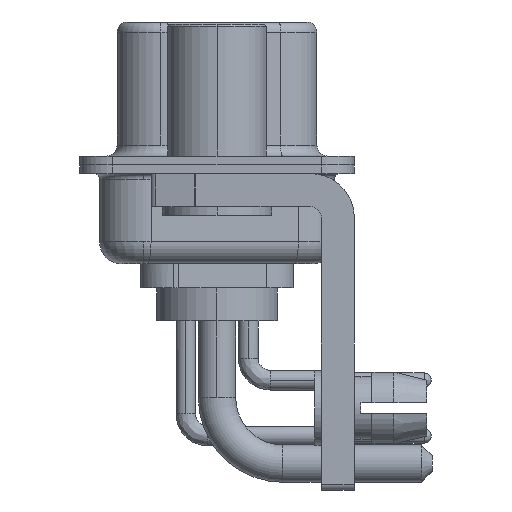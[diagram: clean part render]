
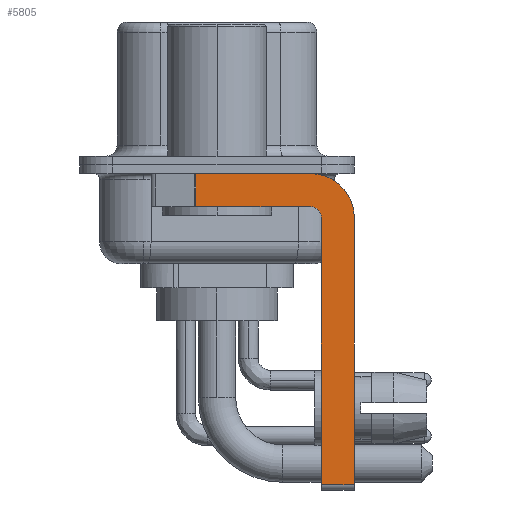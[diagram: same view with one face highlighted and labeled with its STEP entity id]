
A CAD part, left-side view. The second image highlights one B-rep face of the part: STEP entity #5805.
In plain terms, the highlighted planar face has unit normal (-1, 0, 0).
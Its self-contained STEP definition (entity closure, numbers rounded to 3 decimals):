
#283 = CARTESIAN_POINT ( 'NONE',  ( -2.9, -4.25, -1.9 ) ) ;
#370 = AXIS2_PLACEMENT_3D ( 'NONE', #6989, #23847, #5135 ) ;
#701 = EDGE_LOOP ( 'NONE', ( #30869, #20856, #23458, #31140, #3520, #12303, #23858, #1163 ) ) ;
#792 = VECTOR ( 'NONE', #8494, 1000. ) ;
#1113 = LINE ( 'NONE', #6142, #18823 ) ;
#1163 = ORIENTED_EDGE ( 'NONE', *, *, #11047, .F. ) ;
#1188 = AXIS2_PLACEMENT_3D ( 'NONE', #22629, #5762, #15649 ) ;
#1211 = CARTESIAN_POINT ( 'NONE',  ( -2.9, -4.75, -2.4 ) ) ;
#1866 = EDGE_CURVE ( 'NONE', #26353, #20936, #12810, .T. ) ;
#2112 = EDGE_CURVE ( 'NONE', #27599, #7513, #30706, .T. ) ;
#2295 = VECTOR ( 'NONE', #22790, 1000. ) ;
#3507 = VERTEX_POINT ( 'NONE', #7962 ) ;
#3520 = ORIENTED_EDGE ( 'NONE', *, *, #12509, .F. ) ;
#4243 = VERTEX_POINT ( 'NONE', #29832 ) ;
#5135 = DIRECTION ( 'NONE',  ( 0., 0., 1. ) ) ;
#5376 = AXIS2_PLACEMENT_3D ( 'NONE', #12757, #8661, #26011 ) ;
#5597 = CARTESIAN_POINT ( 'NONE',  ( -2.9, -4.25, -0.4 ) ) ;
#5762 = DIRECTION ( 'NONE',  ( 1., 0., 0. ) ) ;
#5805 = ADVANCED_FACE ( 'NONE', ( #27972 ), #24917, .F. ) ;
#6060 = CARTESIAN_POINT ( 'NONE',  ( -2.9, -4.25, -14.55 ) ) ;
#6142 = CARTESIAN_POINT ( 'NONE',  ( -2.9, -4.25, -1.9 ) ) ;
#6989 = CARTESIAN_POINT ( 'NONE',  ( -2.9, -4.25, -2.4 ) ) ;
#7513 = VERTEX_POINT ( 'NONE', #13481 ) ;
#7633 = CARTESIAN_POINT ( 'NONE',  ( -2.9, -6.25, -2.4 ) ) ;
#7962 = CARTESIAN_POINT ( 'NONE',  ( -2.9, 0.978, -0.4 ) ) ;
#8198 = CARTESIAN_POINT ( 'NONE',  ( -2.9, 0.978, -1.9 ) ) ;
#8447 = CARTESIAN_POINT ( 'NONE',  ( -2.9, -4.75, -14.8 ) ) ;
#8494 = DIRECTION ( 'NONE',  ( 0., -1., 0. ) ) ;
#8572 = DIRECTION ( 'NONE',  ( 0., 1., 0. ) ) ;
#8661 = DIRECTION ( 'NONE',  ( 1., 0., 0. ) ) ;
#8987 = VERTEX_POINT ( 'NONE', #7633 ) ;
#9289 = VECTOR ( 'NONE', #19247, 1000. ) ;
#10403 = EDGE_CURVE ( 'NONE', #20936, #4243, #1113, .T. ) ;
#10653 = VECTOR ( 'NONE', #20603, 1000. ) ;
#11047 = EDGE_CURVE ( 'NONE', #27432, #8987, #15217, .T. ) ;
#11790 = LINE ( 'NONE', #31575, #9289 ) ;
#12303 = ORIENTED_EDGE ( 'NONE', *, *, #2112, .T. ) ;
#12509 = EDGE_CURVE ( 'NONE', #27599, #26353, #28067, .T. ) ;
#12757 = CARTESIAN_POINT ( 'NONE',  ( -2.9, -4.25, -2.4 ) ) ;
#12810 = CIRCLE ( 'NONE', #370, 0.5 ) ;
#13481 = CARTESIAN_POINT ( 'NONE',  ( -2.9, -6.25, -14.55 ) ) ;
#13975 = VECTOR ( 'NONE', #21275, 1000. ) ;
#13987 = CARTESIAN_POINT ( 'NONE',  ( -2.9, 3., -0.4 ) ) ;
#15173 = LINE ( 'NONE', #8198, #2295 ) ;
#15217 = CIRCLE ( 'NONE', #5376, 2. ) ;
#15649 = DIRECTION ( 'NONE',  ( 0., 0., -1. ) ) ;
#16253 = LINE ( 'NONE', #13987, #13975 ) ;
#18493 = EDGE_CURVE ( 'NONE', #8987, #7513, #11790, .T. ) ;
#18823 = VECTOR ( 'NONE', #8572, 1000. ) ;
#19247 = DIRECTION ( 'NONE',  ( 0., 0., -1. ) ) ;
#19394 = EDGE_CURVE ( 'NONE', #3507, #27432, #16253, .T. ) ;
#20603 = DIRECTION ( 'NONE',  ( 0., 0., 1. ) ) ;
#20856 = ORIENTED_EDGE ( 'NONE', *, *, #27463, .T. ) ;
#20936 = VERTEX_POINT ( 'NONE', #283 ) ;
#21275 = DIRECTION ( 'NONE',  ( 0., -1., 0. ) ) ;
#22629 = CARTESIAN_POINT ( 'NONE',  ( -2.9, -4.25, -2.4 ) ) ;
#22790 = DIRECTION ( 'NONE',  ( 0., 0., -1. ) ) ;
#23458 = ORIENTED_EDGE ( 'NONE', *, *, #10403, .F. ) ;
#23847 = DIRECTION ( 'NONE',  ( -1., 0., 0. ) ) ;
#23858 = ORIENTED_EDGE ( 'NONE', *, *, #18493, .F. ) ;
#24917 = PLANE ( 'NONE',  #1188 ) ;
#26011 = DIRECTION ( 'NONE',  ( 0., 0., -1. ) ) ;
#26353 = VERTEX_POINT ( 'NONE', #1211 ) ;
#27432 = VERTEX_POINT ( 'NONE', #5597 ) ;
#27463 = EDGE_CURVE ( 'NONE', #3507, #4243, #15173, .T. ) ;
#27599 = VERTEX_POINT ( 'NONE', #28625 ) ;
#27972 = FACE_OUTER_BOUND ( 'NONE', #701, .T. ) ;
#28067 = LINE ( 'NONE', #8447, #10653 ) ;
#28625 = CARTESIAN_POINT ( 'NONE',  ( -2.9, -4.75, -14.55 ) ) ;
#29832 = CARTESIAN_POINT ( 'NONE',  ( -2.9, 0.978, -1.9 ) ) ;
#30706 = LINE ( 'NONE', #6060, #792 ) ;
#30869 = ORIENTED_EDGE ( 'NONE', *, *, #19394, .F. ) ;
#31140 = ORIENTED_EDGE ( 'NONE', *, *, #1866, .F. ) ;
#31575 = CARTESIAN_POINT ( 'NONE',  ( -2.9, -6.25, -2.4 ) ) ;
